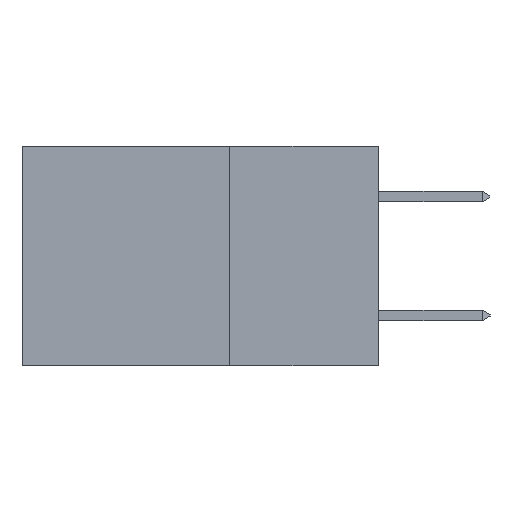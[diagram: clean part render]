
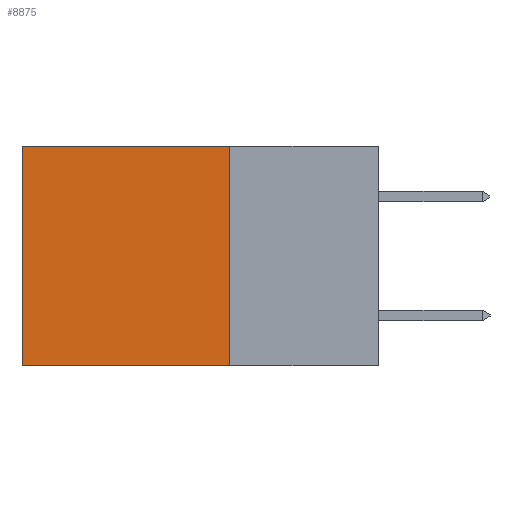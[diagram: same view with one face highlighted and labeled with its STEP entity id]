
A CAD part, left-side view. The second image highlights one B-rep face of the part: STEP entity #8875.
In plain terms, the highlighted planar face has unit normal (-1, 0, 0).
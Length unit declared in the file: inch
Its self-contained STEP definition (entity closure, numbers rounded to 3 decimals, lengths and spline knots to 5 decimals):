
#70 = VECTOR ( 'NONE', #12789, 39.37008 ) ;
#450 = CARTESIAN_POINT ( 'NONE',  ( 0.2615, 0.25, 0. ) ) ;
#539 = LINE ( 'NONE', #8554, #70 ) ;
#866 = EDGE_CURVE ( 'NONE', #10136, #989, #539, .T. ) ;
#989 = VERTEX_POINT ( 'NONE', #11592 ) ;
#1382 = LINE ( 'NONE', #13405, #7804 ) ;
#3178 = FACE_OUTER_BOUND ( 'NONE', #8408, .T. ) ;
#3571 = DIRECTION ( 'NONE',  ( 0., 0., -1. ) ) ;
#3578 = DIRECTION ( 'NONE',  ( 1., 0., 0. ) ) ;
#3694 = CARTESIAN_POINT ( 'NONE',  ( 0.2615, 0.25, -0.37 ) ) ;
#3743 = AXIS2_PLACEMENT_3D ( 'NONE', #3694, #3578, #3571 ) ;
#3744 = PLANE ( 'NONE',  #3743 ) ;
#4516 = CARTESIAN_POINT ( 'NONE',  ( 0.2615, 0.6, 0. ) ) ;
#4918 = EDGE_CURVE ( 'NONE', #989, #11076, #15050, .T. ) ;
#5090 = EDGE_CURVE ( 'NONE', #10136, #8835, #1382, .T. ) ;
#5805 = EDGE_CURVE ( 'NONE', #8835, #11076, #16059, .T. ) ;
#6029 = CARTESIAN_POINT ( 'NONE',  ( 0.2615, 0.6, -0.37 ) ) ;
#6068 = DIRECTION ( 'NONE',  ( 0., 0., -1. ) ) ;
#6479 = ORIENTED_EDGE ( 'NONE', *, *, #5805, .T. ) ;
#6541 = ORIENTED_EDGE ( 'NONE', *, *, #4918, .F. ) ;
#6648 = ORIENTED_EDGE ( 'NONE', *, *, #866, .F. ) ;
#6662 = ORIENTED_EDGE ( 'NONE', *, *, #5090, .T. ) ;
#7804 = VECTOR ( 'NONE', #13288, 39.37008 ) ;
#8408 = EDGE_LOOP ( 'NONE', ( #6479, #6541, #6648, #6662 ) ) ;
#8554 = CARTESIAN_POINT ( 'NONE',  ( 0.2615, 0.25, -0.37 ) ) ;
#8835 = VERTEX_POINT ( 'NONE', #4516 ) ;
#8875 = ADVANCED_FACE ( 'NONE', ( #3178 ), #3744, .F. ) ;
#9890 = VECTOR ( 'NONE', #6068, 39.37008 ) ;
#10136 = VERTEX_POINT ( 'NONE', #450 ) ;
#11076 = VERTEX_POINT ( 'NONE', #14460 ) ;
#11592 = CARTESIAN_POINT ( 'NONE',  ( 0.2615, 0.25, -0.37 ) ) ;
#11923 = VECTOR ( 'NONE', #14861, 39.37008 ) ;
#12789 = DIRECTION ( 'NONE',  ( 0., 0., -1. ) ) ;
#13288 = DIRECTION ( 'NONE',  ( 0., 1., 0. ) ) ;
#13405 = CARTESIAN_POINT ( 'NONE',  ( 0.2615, 0.25, 0. ) ) ;
#14460 = CARTESIAN_POINT ( 'NONE',  ( 0.2615, 0.6, -0.37 ) ) ;
#14861 = DIRECTION ( 'NONE',  ( 0., 1., 0. ) ) ;
#15000 = CARTESIAN_POINT ( 'NONE',  ( 0.2615, 0.25, -0.37 ) ) ;
#15050 = LINE ( 'NONE', #15000, #11923 ) ;
#16059 = LINE ( 'NONE', #6029, #9890 ) ;
